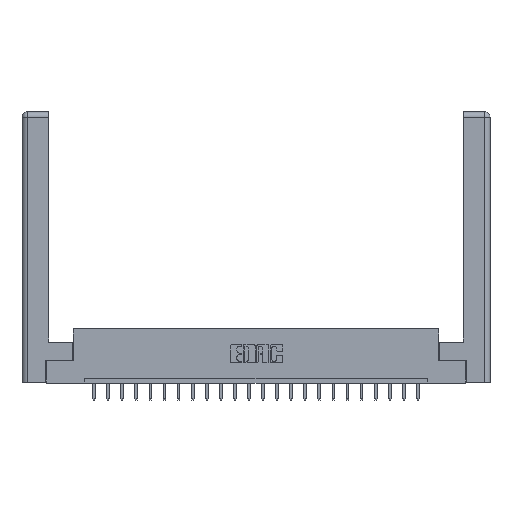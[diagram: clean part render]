
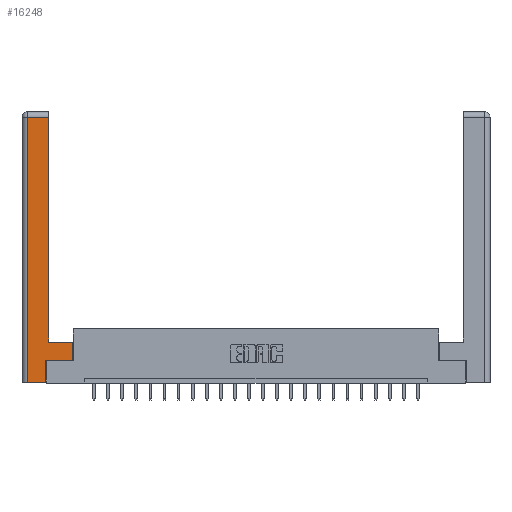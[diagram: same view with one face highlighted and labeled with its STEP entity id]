
A CAD part, top view. The second image highlights one B-rep face of the part: STEP entity #16248.
In plain terms, the highlighted planar face has unit normal (0, 0, 1).
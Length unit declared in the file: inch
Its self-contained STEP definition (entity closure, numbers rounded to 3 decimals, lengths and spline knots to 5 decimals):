
#437 = CARTESIAN_POINT ( 'NONE',  ( 0.295, 3., 0. ) ) ;
#479 = DIRECTION ( 'NONE',  ( -1., 0., 0. ) ) ;
#1172 = DIRECTION ( 'NONE',  ( -1., 0., 0. ) ) ;
#1731 = CARTESIAN_POINT ( 'NONE',  ( 0.265, 0.245, 0. ) ) ;
#1989 = CARTESIAN_POINT ( 'NONE',  ( 0., 0., 0. ) ) ;
#2106 = ORIENTED_EDGE ( 'NONE', *, *, #15077, .T. ) ;
#2370 = ORIENTED_EDGE ( 'NONE', *, *, #11447, .T. ) ;
#2445 = VECTOR ( 'NONE', #12773, 39.37008 ) ;
#2629 = VECTOR ( 'NONE', #17203, 39.37008 ) ;
#3228 = ORIENTED_EDGE ( 'NONE', *, *, #5457, .T. ) ;
#3442 = CARTESIAN_POINT ( 'NONE',  ( 0.565, 0.245, 0. ) ) ;
#4051 = EDGE_CURVE ( 'NONE', #18470, #4822, #12560, .T. ) ;
#4222 = ORIENTED_EDGE ( 'NONE', *, *, #16666, .T. ) ;
#4787 = EDGE_CURVE ( 'NONE', #16587, #15298, #13496, .T. ) ;
#4822 = VERTEX_POINT ( 'NONE', #15838 ) ;
#5285 = CARTESIAN_POINT ( 'NONE',  ( 0.295, 0.45, 0. ) ) ;
#5457 = EDGE_CURVE ( 'NONE', #19084, #19109, #19033, .T. ) ;
#5732 = DIRECTION ( 'NONE',  ( 0., 1., 0. ) ) ;
#5976 = ORIENTED_EDGE ( 'NONE', *, *, #20928, .T. ) ;
#7195 = DIRECTION ( 'NONE',  ( -1., 0., 0. ) ) ;
#7701 = VECTOR ( 'NONE', #8613, 39.37008 ) ;
#8613 = DIRECTION ( 'NONE',  ( 0., 1., 0. ) ) ;
#8633 = CARTESIAN_POINT ( 'NONE',  ( 0.265, 0., 0. ) ) ;
#8777 = VECTOR ( 'NONE', #15755, 39.37008 ) ;
#8860 = CARTESIAN_POINT ( 'NONE',  ( 0.265, 0.245, 0. ) ) ;
#10092 = FACE_OUTER_BOUND ( 'NONE', #21299, .T. ) ;
#10283 = CARTESIAN_POINT ( 'NONE',  ( 0.565, 0.45, 0. ) ) ;
#11245 = CARTESIAN_POINT ( 'NONE',  ( 0.295, 0.45, 0. ) ) ;
#11447 = EDGE_CURVE ( 'NONE', #19109, #18470, #15578, .T. ) ;
#11840 = LINE ( 'NONE', #1731, #7701 ) ;
#11851 = CARTESIAN_POINT ( 'NONE',  ( 0.0615, 2.94, 0. ) ) ;
#11980 = ORIENTED_EDGE ( 'NONE', *, *, #4787, .T. ) ;
#11986 = VECTOR ( 'NONE', #5732, 39.37008 ) ;
#12447 = PLANE ( 'NONE',  #20099 ) ;
#12560 = LINE ( 'NONE', #11851, #15033 ) ;
#12773 = DIRECTION ( 'NONE',  ( 1., 0., 0. ) ) ;
#13130 = CARTESIAN_POINT ( 'NONE',  ( 0.565, 0.45, 0. ) ) ;
#13496 = LINE ( 'NONE', #8633, #8777 ) ;
#13764 = VECTOR ( 'NONE', #479, 39.37008 ) ;
#13884 = CARTESIAN_POINT ( 'NONE',  ( 0.0615, 0., 0. ) ) ;
#14044 = LINE ( 'NONE', #13130, #20662 ) ;
#15033 = VECTOR ( 'NONE', #1172, 39.37008 ) ;
#15077 = EDGE_CURVE ( 'NONE', #15298, #22390, #11840, .T. ) ;
#15176 = CARTESIAN_POINT ( 'NONE',  ( 0.295, 2.94, 0. ) ) ;
#15238 = EDGE_CURVE ( 'NONE', #19653, #19084, #14044, .T. ) ;
#15298 = VERTEX_POINT ( 'NONE', #17382 ) ;
#15578 = LINE ( 'NONE', #437, #11986 ) ;
#15727 = LINE ( 'NONE', #19729, #2445 ) ;
#15755 = DIRECTION ( 'NONE',  ( 1., 0., 0. ) ) ;
#15838 = CARTESIAN_POINT ( 'NONE',  ( 0.0615, 2.94, 0. ) ) ;
#16248 = ADVANCED_FACE ( 'NONE', ( #10092 ), #12447, .F. ) ;
#16587 = VERTEX_POINT ( 'NONE', #18918 ) ;
#16666 = EDGE_CURVE ( 'NONE', #4822, #16587, #21460, .T. ) ;
#17203 = DIRECTION ( 'NONE',  ( 0., -1., 0. ) ) ;
#17382 = CARTESIAN_POINT ( 'NONE',  ( 0.265, 0., 0. ) ) ;
#18470 = VERTEX_POINT ( 'NONE', #15176 ) ;
#18918 = CARTESIAN_POINT ( 'NONE',  ( 0.0615, 0., 0. ) ) ;
#19033 = LINE ( 'NONE', #11245, #13764 ) ;
#19084 = VERTEX_POINT ( 'NONE', #10283 ) ;
#19109 = VERTEX_POINT ( 'NONE', #5285 ) ;
#19272 = ORIENTED_EDGE ( 'NONE', *, *, #4051, .T. ) ;
#19653 = VERTEX_POINT ( 'NONE', #3442 ) ;
#19729 = CARTESIAN_POINT ( 'NONE',  ( 0.565, 0.245, 0. ) ) ;
#20099 = AXIS2_PLACEMENT_3D ( 'NONE', #1989, #21246, #7195 ) ;
#20662 = VECTOR ( 'NONE', #22020, 39.37008 ) ;
#20877 = ORIENTED_EDGE ( 'NONE', *, *, #15238, .T. ) ;
#20928 = EDGE_CURVE ( 'NONE', #22390, #19653, #15727, .T. ) ;
#21246 = DIRECTION ( 'NONE',  ( 0., 0., -1. ) ) ;
#21299 = EDGE_LOOP ( 'NONE', ( #2370, #19272, #4222, #11980, #2106, #5976, #20877, #3228 ) ) ;
#21460 = LINE ( 'NONE', #13884, #2629 ) ;
#22020 = DIRECTION ( 'NONE',  ( 0., 1., 0. ) ) ;
#22390 = VERTEX_POINT ( 'NONE', #8860 ) ;
